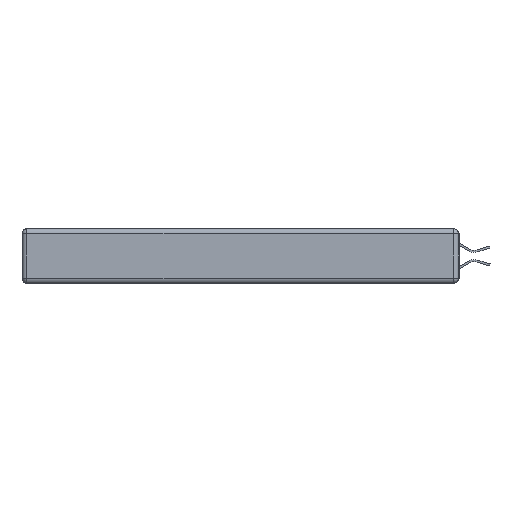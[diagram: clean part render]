
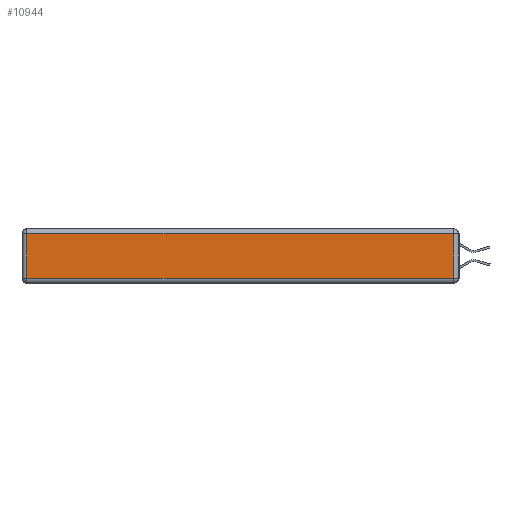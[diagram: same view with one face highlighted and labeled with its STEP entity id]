
A CAD part, left-side view. The second image highlights one B-rep face of the part: STEP entity #10944.
In plain terms, the highlighted planar face has unit normal (-1, 0, 0).
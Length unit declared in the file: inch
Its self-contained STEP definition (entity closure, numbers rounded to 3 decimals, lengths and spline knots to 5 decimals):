
#20 = LINE ( 'NONE', #6051, #14719 ) ;
#1179 = ORIENTED_EDGE ( 'NONE', *, *, #19230, .T. ) ;
#1243 = CARTESIAN_POINT ( 'NONE',  ( 0., 2.72, -0.313 ) ) ;
#1841 = DIRECTION ( 'NONE',  ( 0., 0., -1. ) ) ;
#1883 = CARTESIAN_POINT ( 'NONE',  ( 0., 0.03, -0.03 ) ) ;
#2500 = ORIENTED_EDGE ( 'NONE', *, *, #12837, .T. ) ;
#3312 = LINE ( 'NONE', #12228, #6148 ) ;
#4415 = FACE_OUTER_BOUND ( 'NONE', #6649, .T. ) ;
#4604 = DIRECTION ( 'NONE',  ( 0., 0., 1. ) ) ;
#5163 = CARTESIAN_POINT ( 'NONE',  ( 0., 2.72, -0.03 ) ) ;
#5590 = VERTEX_POINT ( 'NONE', #14184 ) ;
#5598 = CARTESIAN_POINT ( 'NONE',  ( 0., 0., -0.313 ) ) ;
#5687 = LINE ( 'NONE', #13522, #7097 ) ;
#6051 = CARTESIAN_POINT ( 'NONE',  ( 0., 0.03, -0.343 ) ) ;
#6148 = VECTOR ( 'NONE', #1841, 39.37008 ) ;
#6402 = VECTOR ( 'NONE', #17500, 39.37008 ) ;
#6649 = EDGE_LOOP ( 'NONE', ( #13575, #1179, #11416, #2500 ) ) ;
#7097 = VECTOR ( 'NONE', #17698, 39.37008 ) ;
#7289 = VERTEX_POINT ( 'NONE', #1883 ) ;
#10703 = EDGE_CURVE ( 'NONE', #17830, #5590, #12458, .T. ) ;
#10944 = ADVANCED_FACE ( 'NONE', ( #4415 ), #16489, .T. ) ;
#11416 = ORIENTED_EDGE ( 'NONE', *, *, #12547, .T. ) ;
#12132 = CARTESIAN_POINT ( 'NONE',  ( 0., 0., -0.343 ) ) ;
#12228 = CARTESIAN_POINT ( 'NONE',  ( 0., 2.72, -0.343 ) ) ;
#12458 = LINE ( 'NONE', #5598, #6402 ) ;
#12547 = EDGE_CURVE ( 'NONE', #7289, #16350, #5687, .T. ) ;
#12837 = EDGE_CURVE ( 'NONE', #16350, #17830, #3312, .T. ) ;
#13061 = AXIS2_PLACEMENT_3D ( 'NONE', #12132, #19548, #4604 ) ;
#13522 = CARTESIAN_POINT ( 'NONE',  ( 0., 2.75, -0.03 ) ) ;
#13575 = ORIENTED_EDGE ( 'NONE', *, *, #10703, .T. ) ;
#14184 = CARTESIAN_POINT ( 'NONE',  ( 0., 0.03, -0.313 ) ) ;
#14719 = VECTOR ( 'NONE', #16660, 39.37008 ) ;
#16350 = VERTEX_POINT ( 'NONE', #5163 ) ;
#16489 = PLANE ( 'NONE',  #13061 ) ;
#16660 = DIRECTION ( 'NONE',  ( 0., 0., 1. ) ) ;
#17500 = DIRECTION ( 'NONE',  ( 0., -1., 0. ) ) ;
#17698 = DIRECTION ( 'NONE',  ( 0., 1., 0. ) ) ;
#17830 = VERTEX_POINT ( 'NONE', #1243 ) ;
#19230 = EDGE_CURVE ( 'NONE', #5590, #7289, #20, .T. ) ;
#19548 = DIRECTION ( 'NONE',  ( -1., 0., 0. ) ) ;
